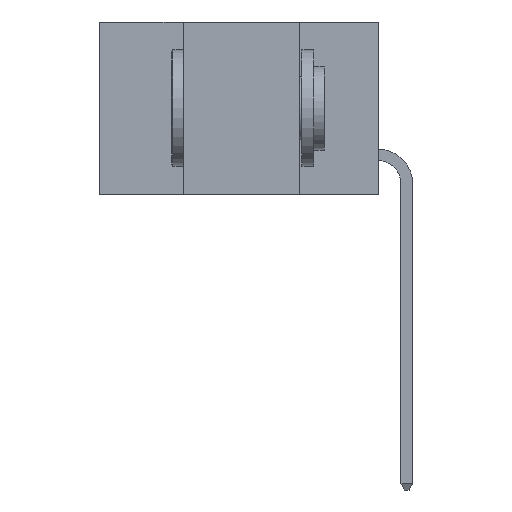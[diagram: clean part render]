
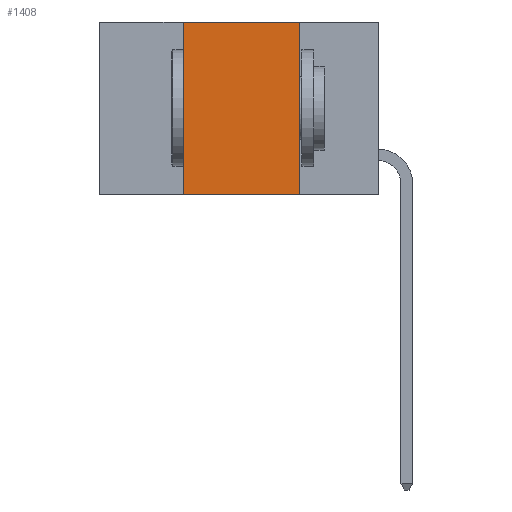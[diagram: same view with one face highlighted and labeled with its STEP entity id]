
A CAD part, left-side view. The second image highlights one B-rep face of the part: STEP entity #1408.
In plain terms, the highlighted planar face has unit normal (-1, 0, 0).
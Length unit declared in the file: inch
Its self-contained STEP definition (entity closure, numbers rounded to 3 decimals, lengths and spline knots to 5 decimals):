
#68 = ORIENTED_EDGE ( 'NONE', *, *, #7052, .T. ) ;
#966 = LINE ( 'NONE', #8750, #5470 ) ;
#1088 = VECTOR ( 'NONE', #9340, 39.37008 ) ;
#1408 = ADVANCED_FACE ( 'NONE', ( #10071 ), #9471, .F. ) ;
#1758 = EDGE_CURVE ( 'NONE', #2001, #5008, #966, .T. ) ;
#1824 = ORIENTED_EDGE ( 'NONE', *, *, #4529, .F. ) ;
#2001 = VERTEX_POINT ( 'NONE', #3724 ) ;
#2025 = VECTOR ( 'NONE', #2652, 39.37008 ) ;
#2378 = CARTESIAN_POINT ( 'NONE',  ( 0., 0.17, -0.37 ) ) ;
#2407 = CARTESIAN_POINT ( 'NONE',  ( 0., 0.17, -0.37 ) ) ;
#2542 = CARTESIAN_POINT ( 'NONE',  ( 0., 0.42, 0. ) ) ;
#2652 = DIRECTION ( 'NONE',  ( 0., -1., 0. ) ) ;
#3084 = LINE ( 'NONE', #8574, #6509 ) ;
#3282 = LINE ( 'NONE', #2407, #1088 ) ;
#3666 = VERTEX_POINT ( 'NONE', #2378 ) ;
#3724 = CARTESIAN_POINT ( 'NONE',  ( 0., 0.42, -0.37 ) ) ;
#4073 = AXIS2_PLACEMENT_3D ( 'NONE', #6832, #9337, #4905 ) ;
#4240 = ORIENTED_EDGE ( 'NONE', *, *, #1758, .F. ) ;
#4529 = EDGE_CURVE ( 'NONE', #5008, #6317, #3084, .T. ) ;
#4905 = DIRECTION ( 'NONE',  ( 0., 0., -1. ) ) ;
#5008 = VERTEX_POINT ( 'NONE', #2542 ) ;
#5027 = CARTESIAN_POINT ( 'NONE',  ( 0., 0.6, -0.37 ) ) ;
#5470 = VECTOR ( 'NONE', #8576, 39.37008 ) ;
#5674 = EDGE_LOOP ( 'NONE', ( #7590, #1824, #4240, #68 ) ) ;
#5993 = LINE ( 'NONE', #5027, #2025 ) ;
#6317 = VERTEX_POINT ( 'NONE', #7232 ) ;
#6400 = DIRECTION ( 'NONE',  ( 0., -1., 0. ) ) ;
#6509 = VECTOR ( 'NONE', #6400, 39.37008 ) ;
#6832 = CARTESIAN_POINT ( 'NONE',  ( 0., 0.6, 0. ) ) ;
#7052 = EDGE_CURVE ( 'NONE', #2001, #3666, #5993, .T. ) ;
#7232 = CARTESIAN_POINT ( 'NONE',  ( 0., 0.17, 0. ) ) ;
#7590 = ORIENTED_EDGE ( 'NONE', *, *, #7716, .F. ) ;
#7716 = EDGE_CURVE ( 'NONE', #6317, #3666, #3282, .T. ) ;
#8574 = CARTESIAN_POINT ( 'NONE',  ( 0., 0.6, 0. ) ) ;
#8576 = DIRECTION ( 'NONE',  ( 0., 0., 1. ) ) ;
#8750 = CARTESIAN_POINT ( 'NONE',  ( 0., 0.42, -0.37 ) ) ;
#9337 = DIRECTION ( 'NONE',  ( 1., 0., 0. ) ) ;
#9340 = DIRECTION ( 'NONE',  ( 0., 0., -1. ) ) ;
#9471 = PLANE ( 'NONE',  #4073 ) ;
#10071 = FACE_OUTER_BOUND ( 'NONE', #5674, .T. ) ;
